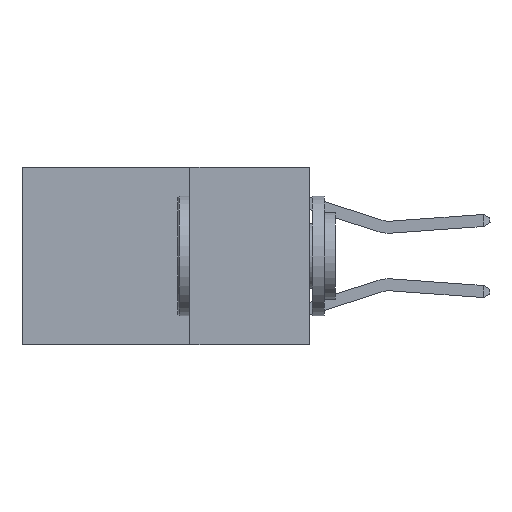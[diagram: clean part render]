
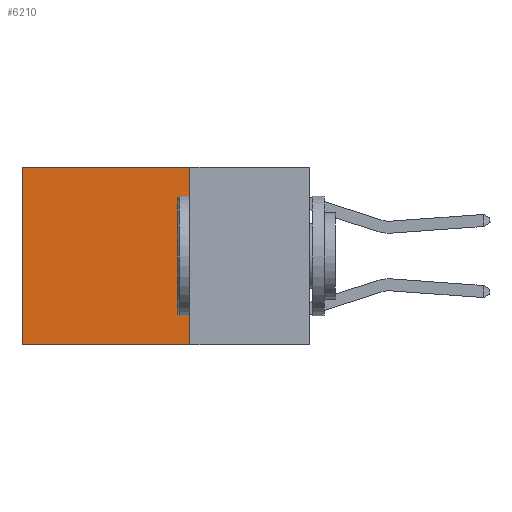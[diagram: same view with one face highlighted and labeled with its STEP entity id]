
A CAD part, left-side view. The second image highlights one B-rep face of the part: STEP entity #6210.
In plain terms, the highlighted planar face has unit normal (-1, 0, 0).
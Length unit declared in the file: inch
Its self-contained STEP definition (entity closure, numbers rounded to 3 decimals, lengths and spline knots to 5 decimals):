
#80 = DIRECTION ( 'NONE',  ( 0., 0., -1. ) ) ;
#343 = EDGE_CURVE ( 'NONE', #1545, #6217, #944, .T. ) ;
#875 = ORIENTED_EDGE ( 'NONE', *, *, #343, .T. ) ;
#944 = LINE ( 'NONE', #8283, #9703 ) ;
#1010 = ORIENTED_EDGE ( 'NONE', *, *, #5789, .F. ) ;
#1086 = VECTOR ( 'NONE', #5490, 39.37008 ) ;
#1545 = VERTEX_POINT ( 'NONE', #9567 ) ;
#1722 = CARTESIAN_POINT ( 'NONE',  ( 0.2625, 0.6, 0. ) ) ;
#1852 = CARTESIAN_POINT ( 'NONE',  ( 0.2625, 0.6, -0.37 ) ) ;
#2199 = ORIENTED_EDGE ( 'NONE', *, *, #8126, .T. ) ;
#3028 = DIRECTION ( 'NONE',  ( 0., 0., -1. ) ) ;
#3362 = LINE ( 'NONE', #4650, #1086 ) ;
#3432 = CARTESIAN_POINT ( 'NONE',  ( 0.2625, 0.25, 0. ) ) ;
#3921 = AXIS2_PLACEMENT_3D ( 'NONE', #3432, #4302, #10178 ) ;
#4135 = VERTEX_POINT ( 'NONE', #7943 ) ;
#4302 = DIRECTION ( 'NONE',  ( 1., 0., 0. ) ) ;
#4650 = CARTESIAN_POINT ( 'NONE',  ( 0.2625, 0.25, -0.37 ) ) ;
#4773 = CARTESIAN_POINT ( 'NONE',  ( 0.2625, 0.25, 0. ) ) ;
#5362 = EDGE_CURVE ( 'NONE', #1545, #4135, #8135, .T. ) ;
#5490 = DIRECTION ( 'NONE',  ( 0., 1., 0. ) ) ;
#5789 = EDGE_CURVE ( 'NONE', #4135, #8533, #3362, .T. ) ;
#5834 = EDGE_LOOP ( 'NONE', ( #2199, #1010, #10504, #875 ) ) ;
#6210 = ADVANCED_FACE ( 'NONE', ( #10611 ), #9334, .F. ) ;
#6217 = VERTEX_POINT ( 'NONE', #1722 ) ;
#6668 = DIRECTION ( 'NONE',  ( 0., 1., 0. ) ) ;
#7943 = CARTESIAN_POINT ( 'NONE',  ( 0.2625, 0.25, -0.37 ) ) ;
#8126 = EDGE_CURVE ( 'NONE', #6217, #8533, #9921, .T. ) ;
#8135 = LINE ( 'NONE', #4773, #10364 ) ;
#8283 = CARTESIAN_POINT ( 'NONE',  ( 0.2625, 0.25, 0. ) ) ;
#8533 = VERTEX_POINT ( 'NONE', #1852 ) ;
#9334 = PLANE ( 'NONE',  #3921 ) ;
#9481 = CARTESIAN_POINT ( 'NONE',  ( 0.2625, 0.6, 0. ) ) ;
#9567 = CARTESIAN_POINT ( 'NONE',  ( 0.2625, 0.25, 0. ) ) ;
#9703 = VECTOR ( 'NONE', #6668, 39.37008 ) ;
#9921 = LINE ( 'NONE', #9481, #11013 ) ;
#10178 = DIRECTION ( 'NONE',  ( 0., 0., -1. ) ) ;
#10364 = VECTOR ( 'NONE', #3028, 39.37008 ) ;
#10504 = ORIENTED_EDGE ( 'NONE', *, *, #5362, .F. ) ;
#10611 = FACE_OUTER_BOUND ( 'NONE', #5834, .T. ) ;
#11013 = VECTOR ( 'NONE', #80, 39.37008 ) ;
